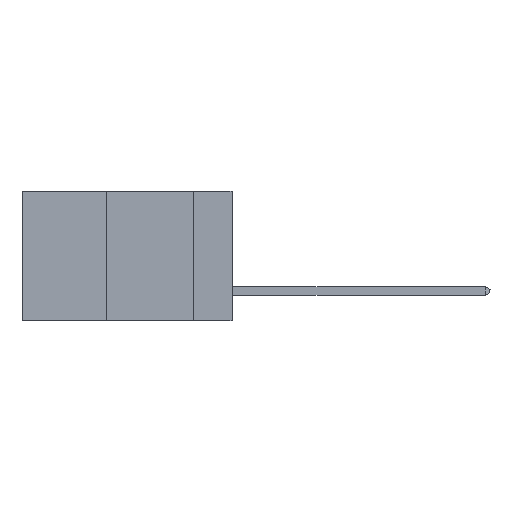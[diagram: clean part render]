
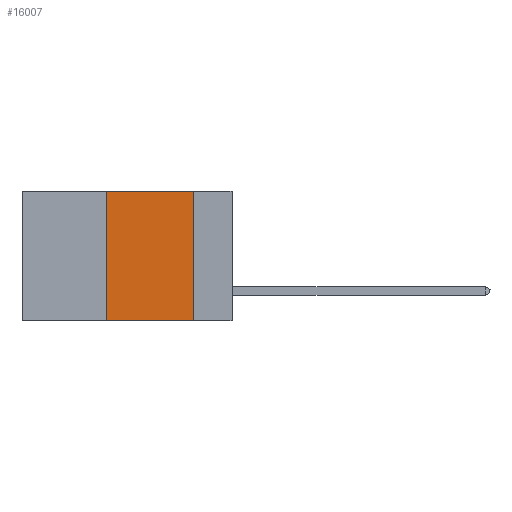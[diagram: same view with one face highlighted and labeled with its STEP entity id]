
A CAD part, left-side view. The second image highlights one B-rep face of the part: STEP entity #16007.
In plain terms, the highlighted planar face has unit normal (-1, 0, 0).
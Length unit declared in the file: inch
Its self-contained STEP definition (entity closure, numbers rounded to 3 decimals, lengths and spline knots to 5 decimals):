
#14 = VERTEX_POINT ( 'NONE', #6727 ) ;
#385 = DIRECTION ( 'NONE',  ( 0., 0., -1. ) ) ;
#1151 = LINE ( 'NONE', #6014, #12575 ) ;
#2762 = EDGE_CURVE ( 'NONE', #14, #5309, #1151, .T. ) ;
#3181 = VERTEX_POINT ( 'NONE', #4111 ) ;
#3964 = DIRECTION ( 'NONE',  ( 0., -1., 0. ) ) ;
#4111 = CARTESIAN_POINT ( 'NONE',  ( 0., 0.36, -0.37 ) ) ;
#4591 = ORIENTED_EDGE ( 'NONE', *, *, #11717, .F. ) ;
#5309 = VERTEX_POINT ( 'NONE', #10180 ) ;
#5431 = VECTOR ( 'NONE', #3964, 39.37008 ) ;
#6014 = CARTESIAN_POINT ( 'NONE',  ( 0., 0.11, 0. ) ) ;
#6727 = CARTESIAN_POINT ( 'NONE',  ( 0., 0.11, 0. ) ) ;
#7620 = DIRECTION ( 'NONE',  ( 0., 0., 1. ) ) ;
#7945 = LINE ( 'NONE', #13010, #11131 ) ;
#7946 = EDGE_CURVE ( 'NONE', #3181, #5309, #10102, .T. ) ;
#8388 = VECTOR ( 'NONE', #9869, 39.37008 ) ;
#9795 = PLANE ( 'NONE',  #12246 ) ;
#9869 = DIRECTION ( 'NONE',  ( 0., -1., 0. ) ) ;
#9924 = CARTESIAN_POINT ( 'NONE',  ( 0., 0.6, 0. ) ) ;
#10031 = CARTESIAN_POINT ( 'NONE',  ( 0., 0.36, 0. ) ) ;
#10102 = LINE ( 'NONE', #17386, #5431 ) ;
#10180 = CARTESIAN_POINT ( 'NONE',  ( 0., 0.11, -0.37 ) ) ;
#10294 = FACE_OUTER_BOUND ( 'NONE', #12947, .T. ) ;
#10550 = VERTEX_POINT ( 'NONE', #10031 ) ;
#11086 = EDGE_CURVE ( 'NONE', #3181, #10550, #7945, .T. ) ;
#11131 = VECTOR ( 'NONE', #7620, 39.37008 ) ;
#11159 = CARTESIAN_POINT ( 'NONE',  ( 0., 0.6, 0. ) ) ;
#11717 = EDGE_CURVE ( 'NONE', #10550, #14, #12177, .T. ) ;
#12094 = ORIENTED_EDGE ( 'NONE', *, *, #2762, .F. ) ;
#12177 = LINE ( 'NONE', #9924, #8388 ) ;
#12246 = AXIS2_PLACEMENT_3D ( 'NONE', #11159, #15255, #385 ) ;
#12575 = VECTOR ( 'NONE', #16960, 39.37008 ) ;
#12947 = EDGE_LOOP ( 'NONE', ( #12094, #4591, #15334, #16158 ) ) ;
#13010 = CARTESIAN_POINT ( 'NONE',  ( 0., 0.36, 0. ) ) ;
#15255 = DIRECTION ( 'NONE',  ( 1., 0., 0. ) ) ;
#15334 = ORIENTED_EDGE ( 'NONE', *, *, #11086, .F. ) ;
#16007 = ADVANCED_FACE ( 'NONE', ( #10294 ), #9795, .F. ) ;
#16158 = ORIENTED_EDGE ( 'NONE', *, *, #7946, .T. ) ;
#16960 = DIRECTION ( 'NONE',  ( 0., 0., -1. ) ) ;
#17386 = CARTESIAN_POINT ( 'NONE',  ( 0., 0.6, -0.37 ) ) ;
